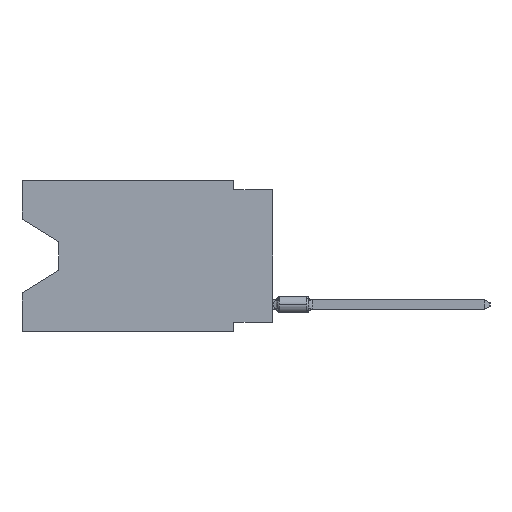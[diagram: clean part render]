
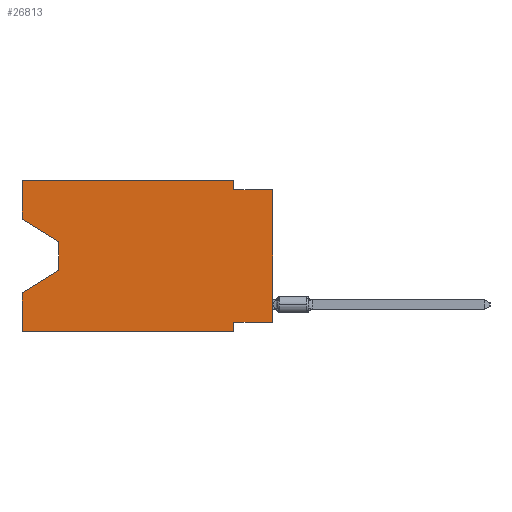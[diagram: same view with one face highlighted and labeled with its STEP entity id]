
A CAD part, left-side view. The second image highlights one B-rep face of the part: STEP entity #26813.
In plain terms, the highlighted planar face has unit normal (-1, 0, 0).
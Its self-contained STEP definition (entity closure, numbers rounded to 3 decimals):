
#1367 = CARTESIAN_POINT ( 'NONE',  ( 0., 2.54, -9.271 ) ) ;
#1416 = DIRECTION ( 'NONE',  ( 0., 0., 1. ) ) ;
#1492 = VERTEX_POINT ( 'NONE', #28688 ) ;
#1548 = CARTESIAN_POINT ( 'NONE',  ( 0., 0., -9.271 ) ) ;
#1808 = EDGE_CURVE ( 'NONE', #13966, #30358, #37460, .T. ) ;
#1917 = VECTOR ( 'NONE', #16869, 1000. ) ;
#2006 = ORIENTED_EDGE ( 'NONE', *, *, #37890, .F. ) ;
#2095 = ORIENTED_EDGE ( 'NONE', *, *, #10636, .T. ) ;
#3641 = EDGE_CURVE ( 'NONE', #13966, #19156, #26710, .T. ) ;
#4698 = CARTESIAN_POINT ( 'NONE',  ( 0., 16.383, -2.546 ) ) ;
#5902 = EDGE_CURVE ( 'NONE', #17709, #19156, #9028, .T. ) ;
#6105 = EDGE_CURVE ( 'NONE', #28717, #30358, #20798, .T. ) ;
#6121 = ORIENTED_EDGE ( 'NONE', *, *, #30911, .F. ) ;
#6647 = CARTESIAN_POINT ( 'NONE',  ( 0., 13.97, -5.893 ) ) ;
#7607 = CARTESIAN_POINT ( 'NONE',  ( 0., 16.383, -9.906 ) ) ;
#7785 = EDGE_CURVE ( 'NONE', #34756, #1492, #28506, .T. ) ;
#8342 = VECTOR ( 'NONE', #30445, 1000. ) ;
#8563 = CARTESIAN_POINT ( 'NONE',  ( 0., 0., -0.635 ) ) ;
#8819 = AXIS2_PLACEMENT_3D ( 'NONE', #10633, #11425, #26164 ) ;
#9028 = LINE ( 'NONE', #6647, #8342 ) ;
#9347 = CARTESIAN_POINT ( 'NONE',  ( 0., 2.54, 0. ) ) ;
#9467 = LINE ( 'NONE', #17771, #16770 ) ;
#10608 = CARTESIAN_POINT ( 'NONE',  ( 0., 16.383, 0. ) ) ;
#10633 = CARTESIAN_POINT ( 'NONE',  ( 0., 16.383, 0. ) ) ;
#10636 = EDGE_CURVE ( 'NONE', #32819, #37170, #25656, .T. ) ;
#11156 = CARTESIAN_POINT ( 'NONE',  ( 0., 2.54, -9.906 ) ) ;
#11425 = DIRECTION ( 'NONE',  ( 1., 0., 0. ) ) ;
#12483 = VECTOR ( 'NONE', #17659, 1000. ) ;
#13634 = EDGE_CURVE ( 'NONE', #23713, #17709, #32134, .T. ) ;
#13966 = VERTEX_POINT ( 'NONE', #30924 ) ;
#15689 = ORIENTED_EDGE ( 'NONE', *, *, #5902, .T. ) ;
#16675 = VERTEX_POINT ( 'NONE', #31964 ) ;
#16770 = VECTOR ( 'NONE', #23850, 1000. ) ;
#16845 = VECTOR ( 'NONE', #34290, 1000. ) ;
#16869 = DIRECTION ( 'NONE',  ( 0., 1., 0. ) ) ;
#17659 = DIRECTION ( 'NONE',  ( 0., 0., -1. ) ) ;
#17709 = VERTEX_POINT ( 'NONE', #37081 ) ;
#17771 = CARTESIAN_POINT ( 'NONE',  ( 0., 16.383, -2.546 ) ) ;
#17939 = CARTESIAN_POINT ( 'NONE',  ( 0., 2.54, -9.906 ) ) ;
#19156 = VERTEX_POINT ( 'NONE', #32692 ) ;
#19753 = ORIENTED_EDGE ( 'NONE', *, *, #1808, .T. ) ;
#20077 = PLANE ( 'NONE',  #8819 ) ;
#20160 = CARTESIAN_POINT ( 'NONE',  ( 0., 13.97, -4.013 ) ) ;
#20778 = ORIENTED_EDGE ( 'NONE', *, *, #27641, .F. ) ;
#20798 = LINE ( 'NONE', #11156, #12483 ) ;
#21008 = VECTOR ( 'NONE', #28602, 1000. ) ;
#21734 = CARTESIAN_POINT ( 'NONE',  ( 0., 0., -0.635 ) ) ;
#22483 = VECTOR ( 'NONE', #24884, 1000. ) ;
#22752 = DIRECTION ( 'NONE',  ( 0., -1., 0. ) ) ;
#23713 = VERTEX_POINT ( 'NONE', #25794 ) ;
#23850 = DIRECTION ( 'NONE',  ( 0., -0.855, -0.519 ) ) ;
#23957 = CARTESIAN_POINT ( 'NONE',  ( 0., 16.383, 0. ) ) ;
#24572 = EDGE_LOOP ( 'NONE', ( #33533, #32382, #15689, #37321, #19753, #31191, #20778, #2095, #6121, #35593, #37204, #2006 ) ) ;
#24694 = DIRECTION ( 'NONE',  ( 0., 0., -1. ) ) ;
#24696 = LINE ( 'NONE', #21734, #22483 ) ;
#24884 = DIRECTION ( 'NONE',  ( 0., -1., 0. ) ) ;
#25656 = LINE ( 'NONE', #34488, #16845 ) ;
#25794 = CARTESIAN_POINT ( 'NONE',  ( 0., 13.97, -4.013 ) ) ;
#26164 = DIRECTION ( 'NONE',  ( 0., 0., -1. ) ) ;
#26710 = LINE ( 'NONE', #23957, #37190 ) ;
#26813 = ADVANCED_FACE ( 'NONE', ( #34991 ), #20077, .F. ) ;
#26904 = DIRECTION ( 'NONE',  ( 0., 0., 1. ) ) ;
#27641 = EDGE_CURVE ( 'NONE', #32819, #28717, #31797, .T. ) ;
#27917 = VECTOR ( 'NONE', #22752, 1000. ) ;
#28506 = LINE ( 'NONE', #10608, #35797 ) ;
#28514 = VECTOR ( 'NONE', #1416, 1000. ) ;
#28602 = DIRECTION ( 'NONE',  ( 0., 0., -1. ) ) ;
#28688 = CARTESIAN_POINT ( 'NONE',  ( 0., 2.54, 0. ) ) ;
#28717 = VERTEX_POINT ( 'NONE', #1367 ) ;
#28816 = VERTEX_POINT ( 'NONE', #4698 ) ;
#30358 = VERTEX_POINT ( 'NONE', #17939 ) ;
#30445 = DIRECTION ( 'NONE',  ( 0., 0.855, -0.519 ) ) ;
#30503 = LINE ( 'NONE', #31265, #28514 ) ;
#30576 = LINE ( 'NONE', #9347, #37394 ) ;
#30911 = EDGE_CURVE ( 'NONE', #16675, #37170, #24696, .T. ) ;
#30924 = CARTESIAN_POINT ( 'NONE',  ( 0., 16.383, -9.906 ) ) ;
#31191 = ORIENTED_EDGE ( 'NONE', *, *, #6105, .F. ) ;
#31265 = CARTESIAN_POINT ( 'NONE',  ( 0., 16.383, 0. ) ) ;
#31741 = CARTESIAN_POINT ( 'NONE',  ( 0., 0., -9.271 ) ) ;
#31797 = LINE ( 'NONE', #1548, #1917 ) ;
#31964 = CARTESIAN_POINT ( 'NONE',  ( 0., 2.54, -0.635 ) ) ;
#32134 = LINE ( 'NONE', #20160, #21008 ) ;
#32382 = ORIENTED_EDGE ( 'NONE', *, *, #13634, .T. ) ;
#32692 = CARTESIAN_POINT ( 'NONE',  ( 0., 16.383, -7.36 ) ) ;
#32819 = VERTEX_POINT ( 'NONE', #31741 ) ;
#33284 = CARTESIAN_POINT ( 'NONE',  ( 0., 16.383, 0. ) ) ;
#33533 = ORIENTED_EDGE ( 'NONE', *, *, #37643, .T. ) ;
#34290 = DIRECTION ( 'NONE',  ( 0., 0., 1. ) ) ;
#34371 = EDGE_CURVE ( 'NONE', #1492, #16675, #30576, .T. ) ;
#34488 = CARTESIAN_POINT ( 'NONE',  ( 0., 0., 0. ) ) ;
#34756 = VERTEX_POINT ( 'NONE', #33284 ) ;
#34991 = FACE_OUTER_BOUND ( 'NONE', #24572, .T. ) ;
#35593 = ORIENTED_EDGE ( 'NONE', *, *, #34371, .F. ) ;
#35797 = VECTOR ( 'NONE', #38503, 1000. ) ;
#37081 = CARTESIAN_POINT ( 'NONE',  ( 0., 13.97, -5.893 ) ) ;
#37170 = VERTEX_POINT ( 'NONE', #8563 ) ;
#37190 = VECTOR ( 'NONE', #26904, 1000. ) ;
#37204 = ORIENTED_EDGE ( 'NONE', *, *, #7785, .F. ) ;
#37321 = ORIENTED_EDGE ( 'NONE', *, *, #3641, .F. ) ;
#37394 = VECTOR ( 'NONE', #24694, 1000. ) ;
#37460 = LINE ( 'NONE', #7607, #27917 ) ;
#37643 = EDGE_CURVE ( 'NONE', #28816, #23713, #9467, .T. ) ;
#37890 = EDGE_CURVE ( 'NONE', #28816, #34756, #30503, .T. ) ;
#38503 = DIRECTION ( 'NONE',  ( 0., -1., 0. ) ) ;
